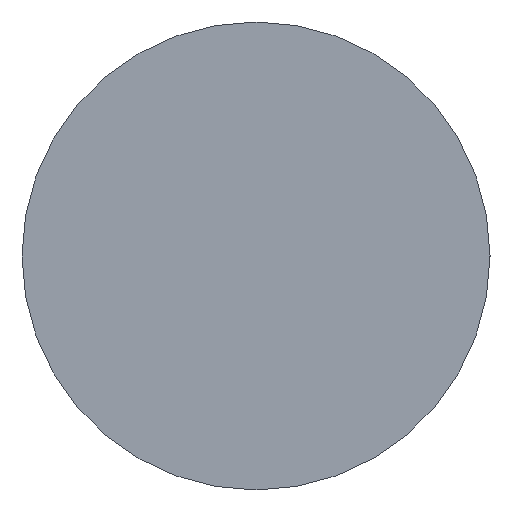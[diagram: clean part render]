
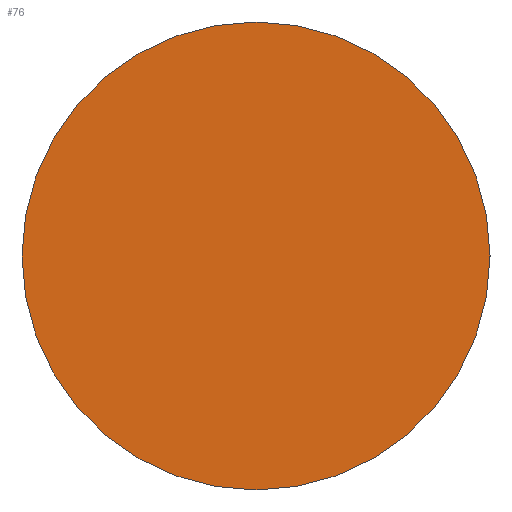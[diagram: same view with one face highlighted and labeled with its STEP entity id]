
A CAD part, left-side view. The second image highlights one B-rep face of the part: STEP entity #76.
In plain terms, the highlighted planar face has unit normal (-1, 0, 0).
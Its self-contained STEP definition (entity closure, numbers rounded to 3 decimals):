
#60 = EDGE_LOOP ( 'NONE', ( #195, #214 ) ) ;
#76 = ADVANCED_FACE ( 'NONE', ( #160 ), #269, .F. ) ;
#150 = CIRCLE ( 'NONE', #190, 5. ) ;
#156 = DIRECTION ( 'NONE',  ( -1., 0., 0. ) ) ;
#160 = FACE_OUTER_BOUND ( 'NONE', #60, .T. ) ;
#189 = VERTEX_POINT ( 'NONE', #438 ) ;
#190 = AXIS2_PLACEMENT_3D ( 'NONE', #339, #336, #334 ) ;
#195 = ORIENTED_EDGE ( 'NONE', *, *, #465, .T. ) ;
#214 = ORIENTED_EDGE ( 'NONE', *, *, #683, .T. ) ;
#269 = PLANE ( 'NONE',  #417 ) ;
#293 = AXIS2_PLACEMENT_3D ( 'NONE', #586, #156, #591 ) ;
#334 = DIRECTION ( 'NONE',  ( 0., 0., 1. ) ) ;
#336 = DIRECTION ( 'NONE',  ( -1., 0., 0. ) ) ;
#339 = CARTESIAN_POINT ( 'NONE',  ( -32.5, 0., 0. ) ) ;
#405 = DIRECTION ( 'NONE',  ( 0., 0., -1. ) ) ;
#407 = DIRECTION ( 'NONE',  ( 1., 0., 0. ) ) ;
#412 = CARTESIAN_POINT ( 'NONE',  ( -32.5, 0., 0. ) ) ;
#417 = AXIS2_PLACEMENT_3D ( 'NONE', #412, #407, #405 ) ;
#438 = CARTESIAN_POINT ( 'NONE',  ( -32.5, 0., 5. ) ) ;
#465 = EDGE_CURVE ( 'NONE', #189, #537, #564, .T. ) ;
#537 = VERTEX_POINT ( 'NONE', #639 ) ;
#564 = CIRCLE ( 'NONE', #293, 5. ) ;
#586 = CARTESIAN_POINT ( 'NONE',  ( -32.5, 0., 0. ) ) ;
#591 = DIRECTION ( 'NONE',  ( 0., 0., 1. ) ) ;
#639 = CARTESIAN_POINT ( 'NONE',  ( -32.5, 0., -5. ) ) ;
#683 = EDGE_CURVE ( 'NONE', #537, #189, #150, .T. ) ;
